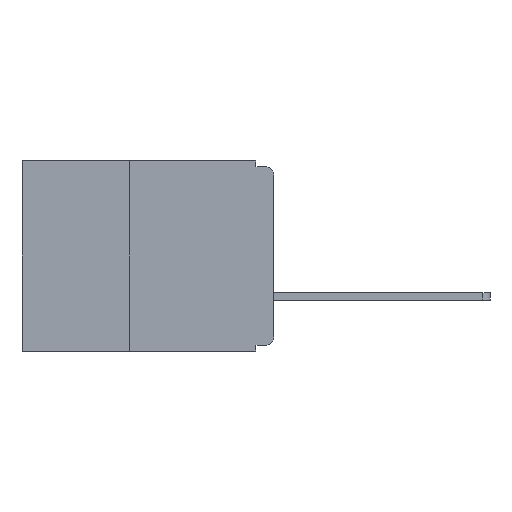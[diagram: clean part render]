
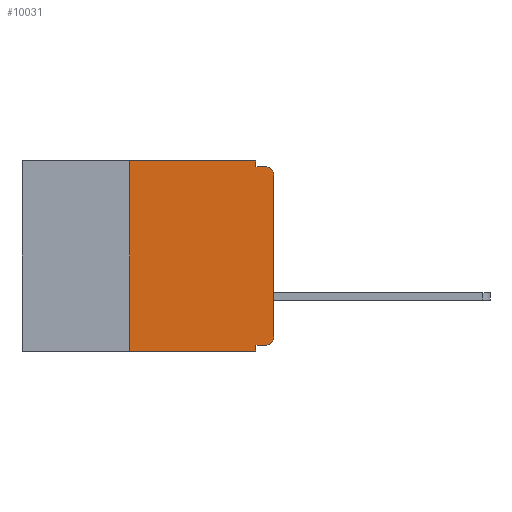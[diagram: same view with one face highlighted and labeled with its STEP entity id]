
A CAD part, left-side view. The second image highlights one B-rep face of the part: STEP entity #10031.
In plain terms, the highlighted planar face has unit normal (-1, 0, 0).
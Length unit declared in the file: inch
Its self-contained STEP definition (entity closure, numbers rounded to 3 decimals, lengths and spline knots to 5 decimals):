
#476 = EDGE_CURVE ( 'NONE', #26915, #30385, #28406, .T. ) ;
#983 = EDGE_CURVE ( 'NONE', #15648, #26097, #23491, .T. ) ;
#1454 = CARTESIAN_POINT ( 'NONE',  ( 0., 0., -0.305 ) ) ;
#1866 = ORIENTED_EDGE ( 'NONE', *, *, #9127, .F. ) ;
#2733 = CARTESIAN_POINT ( 'NONE',  ( 0., 0., -0.01 ) ) ;
#3113 = CARTESIAN_POINT ( 'NONE',  ( 0., 0.437, 0. ) ) ;
#3565 = CARTESIAN_POINT ( 'NONE',  ( 0., 0., 0. ) ) ;
#3918 = DIRECTION ( 'NONE',  ( 0., 0., 1. ) ) ;
#4052 = DIRECTION ( 'NONE',  ( 0., -1., 0. ) ) ;
#4490 = VECTOR ( 'NONE', #3918, 39.37008 ) ;
#4900 = FACE_OUTER_BOUND ( 'NONE', #27234, .T. ) ;
#5871 = DIRECTION ( 'NONE',  ( 0., 0., 1. ) ) ;
#7520 = DIRECTION ( 'NONE',  ( 0., -1., 0. ) ) ;
#7918 = DIRECTION ( 'NONE',  ( 1., 0., 0. ) ) ;
#9127 = EDGE_CURVE ( 'NONE', #26097, #12136, #30160, .T. ) ;
#9411 = VECTOR ( 'NONE', #28076, 39.37008 ) ;
#9603 = EDGE_CURVE ( 'NONE', #23843, #12926, #18356, .T. ) ;
#10021 = VECTOR ( 'NONE', #4052, 39.37008 ) ;
#10031 = ADVANCED_FACE ( 'NONE', ( #4900 ), #24458, .F. ) ;
#10238 = EDGE_CURVE ( 'NONE', #19170, #18898, #17204, .T. ) ;
#10263 = DIRECTION ( 'NONE',  ( 0., 1., 0. ) ) ;
#10301 = CARTESIAN_POINT ( 'NONE',  ( 0., 0., -0.32 ) ) ;
#10762 = LINE ( 'NONE', #27638, #10021 ) ;
#10835 = VECTOR ( 'NONE', #10263, 39.37008 ) ;
#10892 = ORIENTED_EDGE ( 'NONE', *, *, #28130, .T. ) ;
#11138 = AXIS2_PLACEMENT_3D ( 'NONE', #26019, #11807, #28340 ) ;
#11807 = DIRECTION ( 'NONE',  ( -1., 0., 0. ) ) ;
#11947 = CIRCLE ( 'NONE', #11138, 0.015 ) ;
#12136 = VERTEX_POINT ( 'NONE', #12263 ) ;
#12263 = CARTESIAN_POINT ( 'NONE',  ( 0., 0.031, -0.33 ) ) ;
#12926 = VERTEX_POINT ( 'NONE', #15306 ) ;
#13648 = CARTESIAN_POINT ( 'NONE',  ( 0., 0.031, -0.33 ) ) ;
#14080 = VECTOR ( 'NONE', #7520, 39.37008 ) ;
#14109 = VECTOR ( 'NONE', #5871, 39.37008 ) ;
#14272 = AXIS2_PLACEMENT_3D ( 'NONE', #3113, #7918, #24550 ) ;
#15306 = CARTESIAN_POINT ( 'NONE',  ( 0., 0.031, -0.01 ) ) ;
#15648 = VERTEX_POINT ( 'NONE', #16949 ) ;
#16128 = EDGE_CURVE ( 'NONE', #18898, #23843, #16472, .T. ) ;
#16283 = ORIENTED_EDGE ( 'NONE', *, *, #9603, .F. ) ;
#16336 = CARTESIAN_POINT ( 'NONE',  ( 0., 0.25, 0. ) ) ;
#16472 = LINE ( 'NONE', #21079, #9411 ) ;
#16851 = VECTOR ( 'NONE', #24881, 39.37008 ) ;
#16949 = CARTESIAN_POINT ( 'NONE',  ( 0., 0.015, -0.32 ) ) ;
#17204 = LINE ( 'NONE', #20703, #4490 ) ;
#18110 = EDGE_CURVE ( 'NONE', #20359, #26915, #26773, .T. ) ;
#18356 = LINE ( 'NONE', #29439, #16851 ) ;
#18898 = VERTEX_POINT ( 'NONE', #16336 ) ;
#19170 = VERTEX_POINT ( 'NONE', #29625 ) ;
#19652 = ORIENTED_EDGE ( 'NONE', *, *, #983, .F. ) ;
#20263 = ORIENTED_EDGE ( 'NONE', *, *, #18110, .T. ) ;
#20359 = VERTEX_POINT ( 'NONE', #1454 ) ;
#20700 = AXIS2_PLACEMENT_3D ( 'NONE', #25736, #25177, #25303 ) ;
#20703 = CARTESIAN_POINT ( 'NONE',  ( 0., 0.25, -0.33 ) ) ;
#20852 = DIRECTION ( 'NONE',  ( 0., 0., -1. ) ) ;
#21079 = CARTESIAN_POINT ( 'NONE',  ( 0., 0.437, 0. ) ) ;
#21771 = ORIENTED_EDGE ( 'NONE', *, *, #16128, .F. ) ;
#22356 = CARTESIAN_POINT ( 'NONE',  ( 0., 0., -0.025 ) ) ;
#23491 = LINE ( 'NONE', #10301, #10835 ) ;
#23843 = VERTEX_POINT ( 'NONE', #24692 ) ;
#23977 = VECTOR ( 'NONE', #20852, 39.37008 ) ;
#24175 = EDGE_CURVE ( 'NONE', #15648, #20359, #11947, .T. ) ;
#24458 = PLANE ( 'NONE',  #14272 ) ;
#24518 = ORIENTED_EDGE ( 'NONE', *, *, #476, .T. ) ;
#24550 = DIRECTION ( 'NONE',  ( 0., 0., -1. ) ) ;
#24692 = CARTESIAN_POINT ( 'NONE',  ( 0., 0.031, 0. ) ) ;
#24881 = DIRECTION ( 'NONE',  ( 0., 0., -1. ) ) ;
#25177 = DIRECTION ( 'NONE',  ( -1., 0., 0. ) ) ;
#25303 = DIRECTION ( 'NONE',  ( 0., 0., -1. ) ) ;
#25736 = CARTESIAN_POINT ( 'NONE',  ( 0., 0.015, -0.025 ) ) ;
#26019 = CARTESIAN_POINT ( 'NONE',  ( 0., 0.015, -0.305 ) ) ;
#26097 = VERTEX_POINT ( 'NONE', #28443 ) ;
#26747 = LINE ( 'NONE', #2733, #14080 ) ;
#26773 = LINE ( 'NONE', #3565, #14109 ) ;
#26915 = VERTEX_POINT ( 'NONE', #22356 ) ;
#27234 = EDGE_LOOP ( 'NONE', ( #20263, #24518, #28466, #16283, #21771, #28632, #10892, #1866, #19652, #30220 ) ) ;
#27411 = CARTESIAN_POINT ( 'NONE',  ( 0., 0.015, -0.01 ) ) ;
#27638 = CARTESIAN_POINT ( 'NONE',  ( 0., 0.437, -0.33 ) ) ;
#27779 = EDGE_CURVE ( 'NONE', #12926, #30385, #26747, .T. ) ;
#28076 = DIRECTION ( 'NONE',  ( 0., -1., 0. ) ) ;
#28130 = EDGE_CURVE ( 'NONE', #19170, #12136, #10762, .T. ) ;
#28340 = DIRECTION ( 'NONE',  ( 0., 0., -1. ) ) ;
#28406 = CIRCLE ( 'NONE', #20700, 0.015 ) ;
#28443 = CARTESIAN_POINT ( 'NONE',  ( 0., 0.031, -0.32 ) ) ;
#28466 = ORIENTED_EDGE ( 'NONE', *, *, #27779, .F. ) ;
#28632 = ORIENTED_EDGE ( 'NONE', *, *, #10238, .F. ) ;
#29439 = CARTESIAN_POINT ( 'NONE',  ( 0., 0.031, 0. ) ) ;
#29625 = CARTESIAN_POINT ( 'NONE',  ( 0., 0.25, -0.33 ) ) ;
#30160 = LINE ( 'NONE', #13648, #23977 ) ;
#30220 = ORIENTED_EDGE ( 'NONE', *, *, #24175, .T. ) ;
#30385 = VERTEX_POINT ( 'NONE', #27411 ) ;
